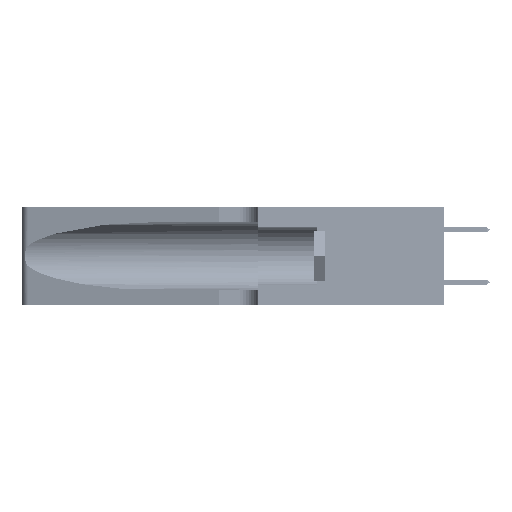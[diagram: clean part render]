
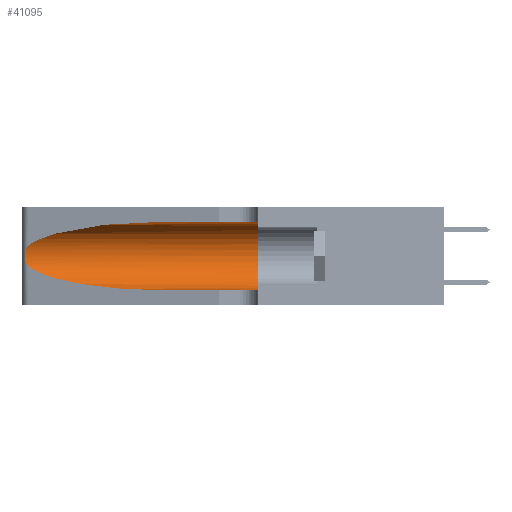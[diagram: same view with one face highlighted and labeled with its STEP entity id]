
A CAD part, left-side view. The second image highlights one B-rep face of the part: STEP entity #41095.
In plain terms, the highlighted cylindrical face has radius 3.308 mm (diameter 6.617 mm), a partial arc.
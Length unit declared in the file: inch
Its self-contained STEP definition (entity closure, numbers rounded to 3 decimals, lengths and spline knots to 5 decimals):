
#2735 = CARTESIAN_POINT ( 'NONE',  ( 0.26075, 1.23896, 0.178 ) ) ;
#2830 = CARTESIAN_POINT ( 'NONE',  ( 0.1305, 0.72297, 0.31525 ) ) ;
#3717 = CYLINDRICAL_SURFACE ( 'NONE', #32584, 0.13025 ) ;
#5618 = ORIENTED_EDGE ( 'NONE', *, *, #26955, .F. ) ;
#6025 = CARTESIAN_POINT ( 'NONE',  ( 0.18966, 0.96281, 0.05475 ) ) ;
#6805 = CARTESIAN_POINT ( 'NONE',  ( 0.25856, 1.23593, 0.16098 ) ) ;
#6881 = CARTESIAN_POINT ( 'NONE',  ( 0.2373, 1.15595, 0.28018 ) ) ;
#6998 = EDGE_CURVE ( 'NONE', #44666, #10352, #15277, .T. ) ;
#7936 = CIRCLE ( 'NONE', #46473, 0.13025 ) ;
#9553 = DIRECTION ( 'NONE',  ( 0., -1., 0. ) ) ;
#9670 = CARTESIAN_POINT ( 'NONE',  ( 0.1305, 0.72297, 0.05475 ) ) ;
#10352 = VERTEX_POINT ( 'NONE', #38442 ) ;
#10654 = CARTESIAN_POINT ( 'NONE',  ( 0.25639, 1.23184, 0.21858 ) ) ;
#10839 = CARTESIAN_POINT ( 'NONE',  ( 0.25639, 1.23186, 0.15144 ) ) ;
#10906 = VECTOR ( 'NONE', #9553, 39.37008 ) ;
#12165 = DIRECTION ( 'NONE',  ( 0., -1., 0. ) ) ;
#13980 = CARTESIAN_POINT ( 'NONE',  ( 0.2373, 1.15595, 0.08982 ) ) ;
#14196 = VERTEX_POINT ( 'NONE', #48623 ) ;
#14316 = EDGE_LOOP ( 'NONE', ( #45361, #28975, #19554, #51731, #23305, #5618 ) ) ;
#14929 = CARTESIAN_POINT ( 'NONE',  ( 0.25487, 1.22718, 0.14631 ) ) ;
#15277 = LINE ( 'NONE', #30396, #24740 ) ;
#16072 = CARTESIAN_POINT ( 'NONE',  ( 0.1305, 1.61858, 0.185 ) ) ;
#16225 = CARTESIAN_POINT ( 'NONE',  ( 0.1305, 0.35, 0.185 ) ) ;
#16813 = EDGE_CURVE ( 'NONE', #25792, #31694, #30625, .T. ) ;
#18841 = CARTESIAN_POINT ( 'NONE',  ( 0.25487, 1.22718, 0.22369 ) ) ;
#19554 = ORIENTED_EDGE ( 'NONE', *, *, #20721, .T. ) ;
#20324 = DIRECTION ( 'NONE',  ( 0., 0., 1. ) ) ;
#20721 = EDGE_CURVE ( 'NONE', #31694, #44666, #21329, .T. ) ;
#21329 =( BOUNDED_CURVE ( )  B_SPLINE_CURVE ( 3, ( #46102, #13980, #6025, #34267 ),
 .UNSPECIFIED., .F., .F. ) 
 B_SPLINE_CURVE_WITH_KNOTS ( ( 4, 4 ),
 ( 3.44316, 4.71239 ),
 .UNSPECIFIED. ) 
 CURVE ( )  GEOMETRIC_REPRESENTATION_ITEM ( )  RATIONAL_B_SPLINE_CURVE ( ( 1., 0.87, 0.87, 1. ) ) 
 REPRESENTATION_ITEM ( '' )  );
#21694 = LINE ( 'NONE', #29701, #10906 ) ;
#22863 = CARTESIAN_POINT ( 'NONE',  ( 0.25854, 1.2359, 0.20912 ) ) ;
#23305 = ORIENTED_EDGE ( 'NONE', *, *, #42987, .F. ) ;
#24740 = VECTOR ( 'NONE', #50531, 39.37008 ) ;
#25792 = VERTEX_POINT ( 'NONE', #34739 ) ;
#26446 = FACE_OUTER_BOUND ( 'NONE', #14316, .T. ) ;
#26927 = CARTESIAN_POINT ( 'NONE',  ( 0.26075, 1.23896, 0.19203 ) ) ;
#26955 = EDGE_CURVE ( 'NONE', #14196, #47343, #21694, .T. ) ;
#28975 = ORIENTED_EDGE ( 'NONE', *, *, #16813, .T. ) ;
#29556 = CARTESIAN_POINT ( 'NONE',  ( 0.1305, 0.35, 0.31525 ) ) ;
#29701 = CARTESIAN_POINT ( 'NONE',  ( 0.1305, 1.61858, 0.31525 ) ) ;
#29978 =( BOUNDED_CURVE ( )  B_SPLINE_CURVE ( 3, ( #2830, #31077, #6881, #35133 ),
 .UNSPECIFIED., .F., .T. ) 
 B_SPLINE_CURVE_WITH_KNOTS ( ( 4, 4 ),
 ( 1.5708, 2.84003 ),
 .UNSPECIFIED. ) 
 CURVE ( )  GEOMETRIC_REPRESENTATION_ITEM ( )  RATIONAL_B_SPLINE_CURVE ( ( 1., 0.87, 0.87, 1. ) ) 
 REPRESENTATION_ITEM ( '' )  );
#30396 = CARTESIAN_POINT ( 'NONE',  ( 0.1305, 1.61858, 0.05475 ) ) ;
#30625 = B_SPLINE_CURVE_WITH_KNOTS ( 'NONE', 3,
 ( #18841, #42942, #10654, #47044, #22863, #51109, #26927, #2735, #30979, #6805, #35035, #10839, #39103, #14929 ),
 .UNSPECIFIED., .F., .F.,
 ( 4, 2, 2, 2, 2, 2, 4 ),
 ( 0., 0.00027, 0.00053, 0.00107, 0.0016, 0.00187, 0.00214 ),
 .UNSPECIFIED. ) ;
#30979 = CARTESIAN_POINT ( 'NONE',  ( 0.26017, 1.23833, 0.17102 ) ) ;
#31077 = CARTESIAN_POINT ( 'NONE',  ( 0.18966, 0.96281, 0.31525 ) ) ;
#31694 = VERTEX_POINT ( 'NONE', #48421 ) ;
#32584 = AXIS2_PLACEMENT_3D ( 'NONE', #16072, #12165, #48541 ) ;
#34267 = CARTESIAN_POINT ( 'NONE',  ( 0.1305, 0.72297, 0.05475 ) ) ;
#34739 = CARTESIAN_POINT ( 'NONE',  ( 0.25487, 1.22718, 0.22369 ) ) ;
#35035 = CARTESIAN_POINT ( 'NONE',  ( 0.25789, 1.23486, 0.15765 ) ) ;
#35133 = CARTESIAN_POINT ( 'NONE',  ( 0.25487, 1.22718, 0.22369 ) ) ;
#37903 = EDGE_CURVE ( 'NONE', #14196, #25792, #29978, .T. ) ;
#38442 = CARTESIAN_POINT ( 'NONE',  ( 0.1305, 0.35, 0.05475 ) ) ;
#39103 = CARTESIAN_POINT ( 'NONE',  ( 0.25555, 1.22993, 0.14849 ) ) ;
#41095 = ADVANCED_FACE ( 'NONE', ( #26446 ), #3717, .F. ) ;
#42942 = CARTESIAN_POINT ( 'NONE',  ( 0.25555, 1.22994, 0.2215 ) ) ;
#42987 = EDGE_CURVE ( 'NONE', #47343, #10352, #7936, .T. ) ;
#44424 = DIRECTION ( 'NONE',  ( 0., 1., 0. ) ) ;
#44666 = VERTEX_POINT ( 'NONE', #9670 ) ;
#45361 = ORIENTED_EDGE ( 'NONE', *, *, #37903, .T. ) ;
#46102 = CARTESIAN_POINT ( 'NONE',  ( 0.25487, 1.22718, 0.14631 ) ) ;
#46473 = AXIS2_PLACEMENT_3D ( 'NONE', #16225, #44424, #20324 ) ;
#47044 = CARTESIAN_POINT ( 'NONE',  ( 0.25787, 1.23484, 0.2124 ) ) ;
#47343 = VERTEX_POINT ( 'NONE', #29556 ) ;
#48421 = CARTESIAN_POINT ( 'NONE',  ( 0.25487, 1.22718, 0.14631 ) ) ;
#48541 = DIRECTION ( 'NONE',  ( 0., 0., -1. ) ) ;
#48623 = CARTESIAN_POINT ( 'NONE',  ( 0.1305, 0.72297, 0.31525 ) ) ;
#50531 = DIRECTION ( 'NONE',  ( 0., -1., 0. ) ) ;
#51109 = CARTESIAN_POINT ( 'NONE',  ( 0.26018, 1.23835, 0.19895 ) ) ;
#51731 = ORIENTED_EDGE ( 'NONE', *, *, #6998, .T. ) ;
